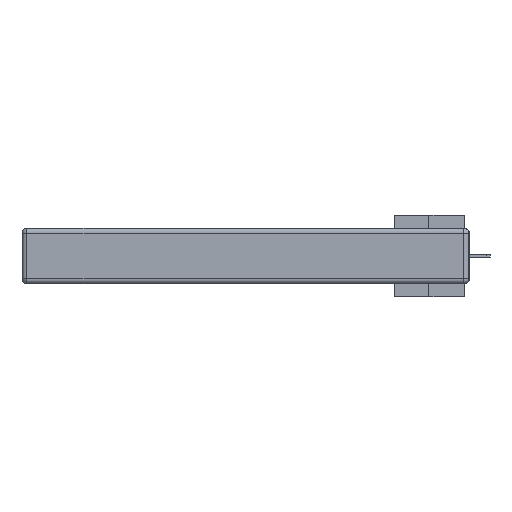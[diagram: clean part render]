
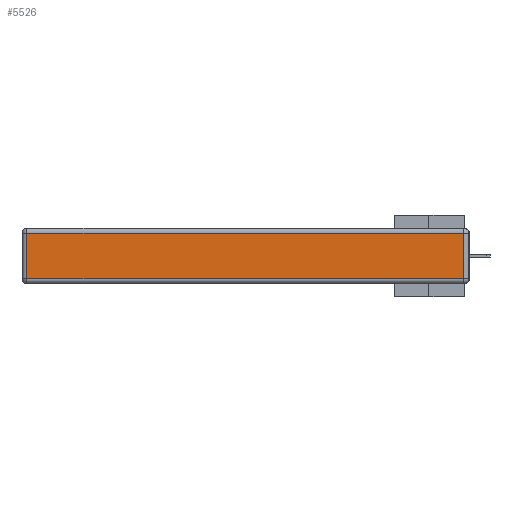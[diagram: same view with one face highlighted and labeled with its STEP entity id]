
A CAD part, left-side view. The second image highlights one B-rep face of the part: STEP entity #5526.
In plain terms, the highlighted planar face has unit normal (-1, 0, 0).
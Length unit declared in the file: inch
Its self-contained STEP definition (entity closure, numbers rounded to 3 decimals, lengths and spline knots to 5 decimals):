
#1673 = ORIENTED_EDGE ( 'NONE', *, *, #9577, .T. ) ;
#2077 = CARTESIAN_POINT ( 'NONE',  ( 0., 0., -0.343 ) ) ;
#3346 = EDGE_CURVE ( 'NONE', #16751, #18951, #6872, .T. ) ;
#3614 = LINE ( 'NONE', #14593, #28551 ) ;
#3984 = EDGE_CURVE ( 'NONE', #27058, #16751, #14486, .T. ) ;
#4008 = VECTOR ( 'NONE', #30900, 39.37008 ) ;
#4499 = DIRECTION ( 'NONE',  ( 0., -1., 0. ) ) ;
#4815 = DIRECTION ( 'NONE',  ( 0., 0., 1. ) ) ;
#5004 = CARTESIAN_POINT ( 'NONE',  ( 0., 2.72, -0.03 ) ) ;
#5526 = ADVANCED_FACE ( 'NONE', ( #19601 ), #9605, .T. ) ;
#6087 = VECTOR ( 'NONE', #4499, 39.37008 ) ;
#6872 = LINE ( 'NONE', #16570, #6087 ) ;
#7433 = AXIS2_PLACEMENT_3D ( 'NONE', #2077, #26390, #12054 ) ;
#8065 = ORIENTED_EDGE ( 'NONE', *, *, #3346, .T. ) ;
#9577 = EDGE_CURVE ( 'NONE', #12022, #27058, #29670, .T. ) ;
#9605 = PLANE ( 'NONE',  #7433 ) ;
#12022 = VERTEX_POINT ( 'NONE', #12962 ) ;
#12054 = DIRECTION ( 'NONE',  ( 0., 0., 1. ) ) ;
#12962 = CARTESIAN_POINT ( 'NONE',  ( 0., 0.03, -0.03 ) ) ;
#14486 = LINE ( 'NONE', #18819, #26433 ) ;
#14593 = CARTESIAN_POINT ( 'NONE',  ( 0., 0.03, -0.343 ) ) ;
#16535 = DIRECTION ( 'NONE',  ( 0., 0., -1. ) ) ;
#16570 = CARTESIAN_POINT ( 'NONE',  ( 0., 0., -0.313 ) ) ;
#16751 = VERTEX_POINT ( 'NONE', #19429 ) ;
#18509 = EDGE_LOOP ( 'NONE', ( #8065, #24798, #1673, #27510 ) ) ;
#18819 = CARTESIAN_POINT ( 'NONE',  ( 0., 2.72, -0.343 ) ) ;
#18951 = VERTEX_POINT ( 'NONE', #20972 ) ;
#19429 = CARTESIAN_POINT ( 'NONE',  ( 0., 2.72, -0.313 ) ) ;
#19601 = FACE_OUTER_BOUND ( 'NONE', #18509, .T. ) ;
#20972 = CARTESIAN_POINT ( 'NONE',  ( 0., 0.03, -0.313 ) ) ;
#24798 = ORIENTED_EDGE ( 'NONE', *, *, #29026, .T. ) ;
#26390 = DIRECTION ( 'NONE',  ( -1., 0., 0. ) ) ;
#26433 = VECTOR ( 'NONE', #16535, 39.37008 ) ;
#27058 = VERTEX_POINT ( 'NONE', #5004 ) ;
#27510 = ORIENTED_EDGE ( 'NONE', *, *, #3984, .T. ) ;
#28551 = VECTOR ( 'NONE', #4815, 39.37008 ) ;
#28637 = CARTESIAN_POINT ( 'NONE',  ( 0., 2.75, -0.03 ) ) ;
#29026 = EDGE_CURVE ( 'NONE', #18951, #12022, #3614, .T. ) ;
#29670 = LINE ( 'NONE', #28637, #4008 ) ;
#30900 = DIRECTION ( 'NONE',  ( 0., 1., 0. ) ) ;
